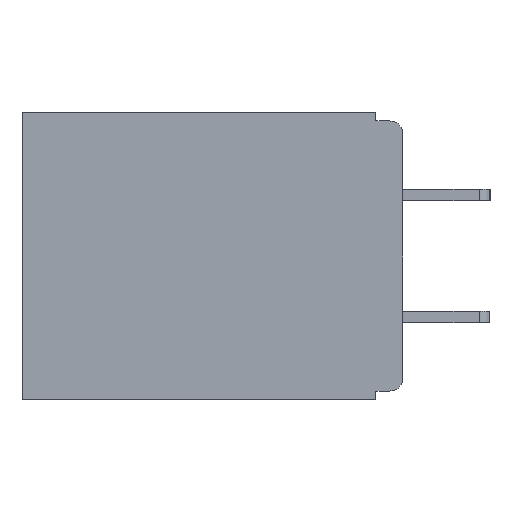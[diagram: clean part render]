
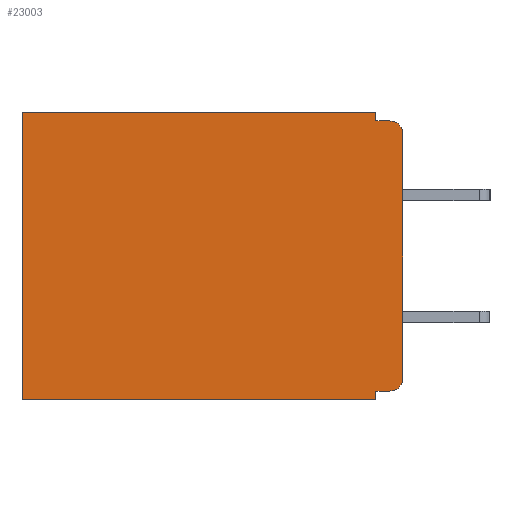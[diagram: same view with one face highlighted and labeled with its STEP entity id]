
A CAD part, left-side view. The second image highlights one B-rep face of the part: STEP entity #23003.
In plain terms, the highlighted planar face has unit normal (-1, 0, 0).
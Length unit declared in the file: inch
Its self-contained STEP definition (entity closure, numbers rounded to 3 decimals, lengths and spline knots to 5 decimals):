
#250 = LINE ( 'NONE', #11484, #25283 ) ;
#1120 = DIRECTION ( 'NONE',  ( 1., 0., 0. ) ) ;
#1261 = DIRECTION ( 'NONE',  ( 0., 1., 0. ) ) ;
#1416 = VERTEX_POINT ( 'NONE', #9183 ) ;
#1604 = FACE_OUTER_BOUND ( 'NONE', #17007, .T. ) ;
#1640 = CARTESIAN_POINT ( 'NONE',  ( 0.3, 0.031, 0. ) ) ;
#1730 = DIRECTION ( 'NONE',  ( 0., 1., 0. ) ) ;
#1779 = AXIS2_PLACEMENT_3D ( 'NONE', #2626, #3064, #3585 ) ;
#2094 = LINE ( 'NONE', #23042, #13876 ) ;
#2626 = CARTESIAN_POINT ( 'NONE',  ( 0.3, 0.015, -0.025 ) ) ;
#3064 = DIRECTION ( 'NONE',  ( -1., 0., 0. ) ) ;
#3544 = VERTEX_POINT ( 'NONE', #22777 ) ;
#3562 = EDGE_CURVE ( 'NONE', #14948, #15588, #20431, .T. ) ;
#3585 = DIRECTION ( 'NONE',  ( 0., 0., -1. ) ) ;
#5476 = CARTESIAN_POINT ( 'NONE',  ( 0.3, 0.031, -0.01 ) ) ;
#5678 = LINE ( 'NONE', #28429, #31302 ) ;
#5883 = CARTESIAN_POINT ( 'NONE',  ( 0.3, 0., -0.305 ) ) ;
#6268 = VECTOR ( 'NONE', #29808, 39.37008 ) ;
#7467 = CARTESIAN_POINT ( 'NONE',  ( 0.3, 0.437, -0.33 ) ) ;
#8132 = EDGE_CURVE ( 'NONE', #19916, #18402, #10789, .T. ) ;
#8143 = VECTOR ( 'NONE', #16728, 39.37008 ) ;
#8160 = DIRECTION ( 'NONE',  ( 0., 0., -1. ) ) ;
#8648 = CARTESIAN_POINT ( 'NONE',  ( 0.3, 0.031, -0.33 ) ) ;
#8960 = EDGE_CURVE ( 'NONE', #14948, #18402, #2094, .T. ) ;
#9183 = CARTESIAN_POINT ( 'NONE',  ( 0.3, 0.031, -0.32 ) ) ;
#9248 = CARTESIAN_POINT ( 'NONE',  ( 0.3, 0., -0.025 ) ) ;
#9269 = CARTESIAN_POINT ( 'NONE',  ( 0.3, 0., -0.32 ) ) ;
#9905 = VERTEX_POINT ( 'NONE', #8648 ) ;
#10650 = ORIENTED_EDGE ( 'NONE', *, *, #30129, .T. ) ;
#10653 = ORIENTED_EDGE ( 'NONE', *, *, #8960, .F. ) ;
#10789 = CIRCLE ( 'NONE', #16630, 0.015 ) ;
#10901 = VERTEX_POINT ( 'NONE', #17971 ) ;
#11484 = CARTESIAN_POINT ( 'NONE',  ( 0.3, 0.031, -0.33 ) ) ;
#12430 = CARTESIAN_POINT ( 'NONE',  ( 0.3, 0.015, -0.305 ) ) ;
#13648 = PLANE ( 'NONE',  #13864 ) ;
#13858 = CARTESIAN_POINT ( 'NONE',  ( 0.3, 0.015, -0.01 ) ) ;
#13864 = AXIS2_PLACEMENT_3D ( 'NONE', #23529, #1120, #18711 ) ;
#13876 = VECTOR ( 'NONE', #8160, 39.37008 ) ;
#13985 = LINE ( 'NONE', #9269, #19848 ) ;
#14948 = VERTEX_POINT ( 'NONE', #9248 ) ;
#14983 = DIRECTION ( 'NONE',  ( 0., 0., -1. ) ) ;
#15588 = VERTEX_POINT ( 'NONE', #13858 ) ;
#16630 = AXIS2_PLACEMENT_3D ( 'NONE', #12430, #29756, #14983 ) ;
#16728 = DIRECTION ( 'NONE',  ( 0., -1., 0. ) ) ;
#16769 = CARTESIAN_POINT ( 'NONE',  ( 0.3, 0.437, 0. ) ) ;
#17007 = EDGE_LOOP ( 'NONE', ( #10653, #24391, #20858, #18415, #10650, #18513, #31546, #26594, #29679, #24668 ) ) ;
#17971 = CARTESIAN_POINT ( 'NONE',  ( 0.3, 0.437, -0.33 ) ) ;
#18402 = VERTEX_POINT ( 'NONE', #5883 ) ;
#18409 = VECTOR ( 'NONE', #21647, 39.37008 ) ;
#18415 = ORIENTED_EDGE ( 'NONE', *, *, #27365, .F. ) ;
#18492 = EDGE_CURVE ( 'NONE', #9905, #10901, #27737, .T. ) ;
#18513 = ORIENTED_EDGE ( 'NONE', *, *, #20015, .T. ) ;
#18532 = DIRECTION ( 'NONE',  ( 0., 1., 0. ) ) ;
#18711 = DIRECTION ( 'NONE',  ( 0., 0., -1. ) ) ;
#19195 = LINE ( 'NONE', #1640, #18409 ) ;
#19713 = CARTESIAN_POINT ( 'NONE',  ( 0.3, 0.015, -0.32 ) ) ;
#19848 = VECTOR ( 'NONE', #1730, 39.37008 ) ;
#19916 = VERTEX_POINT ( 'NONE', #19713 ) ;
#20015 = EDGE_CURVE ( 'NONE', #26281, #10901, #26114, .T. ) ;
#20431 = CIRCLE ( 'NONE', #1779, 0.015 ) ;
#20858 = ORIENTED_EDGE ( 'NONE', *, *, #29613, .F. ) ;
#21277 = CARTESIAN_POINT ( 'NONE',  ( 0.3, 0., -0.33 ) ) ;
#21647 = DIRECTION ( 'NONE',  ( 0., 0., -1. ) ) ;
#22777 = CARTESIAN_POINT ( 'NONE',  ( 0.3, 0.031, 0. ) ) ;
#23003 = ADVANCED_FACE ( 'NONE', ( #1604 ), #13648, .F. ) ;
#23042 = CARTESIAN_POINT ( 'NONE',  ( 0.3, 0., -0.33 ) ) ;
#23529 = CARTESIAN_POINT ( 'NONE',  ( 0.3, 0., -0.33 ) ) ;
#24391 = ORIENTED_EDGE ( 'NONE', *, *, #3562, .T. ) ;
#24668 = ORIENTED_EDGE ( 'NONE', *, *, #8132, .T. ) ;
#25283 = VECTOR ( 'NONE', #26459, 39.37008 ) ;
#25304 = VERTEX_POINT ( 'NONE', #5476 ) ;
#25404 = VECTOR ( 'NONE', #1261, 39.37008 ) ;
#25645 = EDGE_CURVE ( 'NONE', #19916, #1416, #13985, .T. ) ;
#26114 = LINE ( 'NONE', #7467, #6268 ) ;
#26281 = VERTEX_POINT ( 'NONE', #16769 ) ;
#26459 = DIRECTION ( 'NONE',  ( 0., 0., -1. ) ) ;
#26594 = ORIENTED_EDGE ( 'NONE', *, *, #27995, .F. ) ;
#27365 = EDGE_CURVE ( 'NONE', #3544, #25304, #19195, .T. ) ;
#27737 = LINE ( 'NONE', #21277, #25404 ) ;
#27929 = LINE ( 'NONE', #28991, #8143 ) ;
#27995 = EDGE_CURVE ( 'NONE', #1416, #9905, #250, .T. ) ;
#28429 = CARTESIAN_POINT ( 'NONE',  ( 0.3, 0., 0. ) ) ;
#28991 = CARTESIAN_POINT ( 'NONE',  ( 0.3, 0., -0.01 ) ) ;
#29613 = EDGE_CURVE ( 'NONE', #25304, #15588, #27929, .T. ) ;
#29679 = ORIENTED_EDGE ( 'NONE', *, *, #25645, .F. ) ;
#29756 = DIRECTION ( 'NONE',  ( -1., 0., 0. ) ) ;
#29808 = DIRECTION ( 'NONE',  ( 0., 0., -1. ) ) ;
#30129 = EDGE_CURVE ( 'NONE', #3544, #26281, #5678, .T. ) ;
#31302 = VECTOR ( 'NONE', #18532, 39.37008 ) ;
#31546 = ORIENTED_EDGE ( 'NONE', *, *, #18492, .F. ) ;
